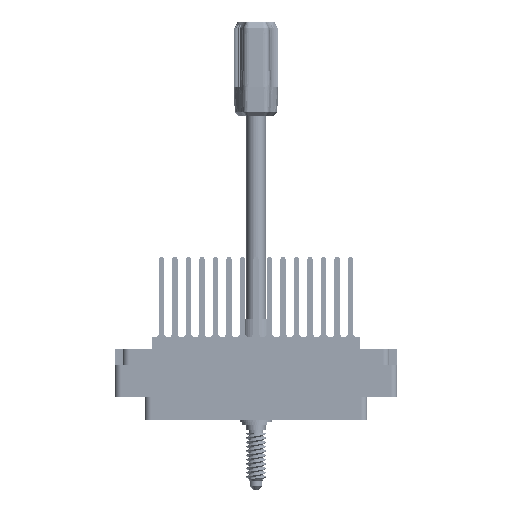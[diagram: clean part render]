
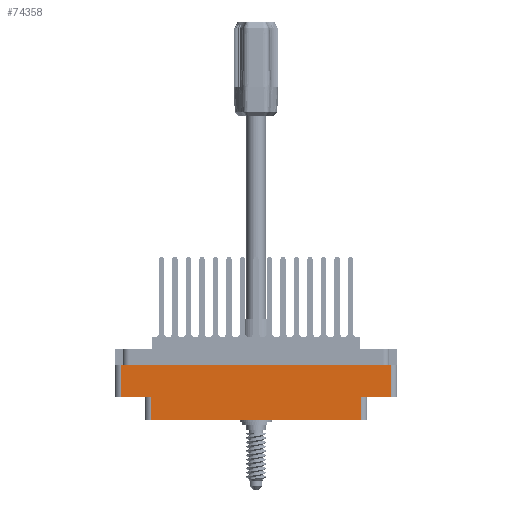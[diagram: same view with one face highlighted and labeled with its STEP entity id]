
A CAD part, front view. The second image highlights one B-rep face of the part: STEP entity #74358.
In plain terms, the highlighted planar face has unit normal (0, -1, 0).
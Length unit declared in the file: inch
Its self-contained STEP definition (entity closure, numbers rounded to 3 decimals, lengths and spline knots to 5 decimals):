
#1422 = CARTESIAN_POINT ( 'NONE',  ( -1.359, -0.617, -0.798 ) ) ;
#1529 = CARTESIAN_POINT ( 'NONE',  ( -1.359, -0.617, -0.798 ) ) ;
#1638 = CARTESIAN_POINT ( 'NONE',  ( 1.297, -0.617, -0.274 ) ) ;
#1776 = CARTESIAN_POINT ( 'NONE',  ( -1.297, -0.617, -0.274 ) ) ;
#3254 = ORIENTED_EDGE ( 'NONE', *, *, #56275, .T. ) ;
#5570 = DIRECTION ( 'NONE',  ( 1., 0., 0. ) ) ;
#8130 = LINE ( 'NONE', #80996, #48906 ) ;
#8278 = CARTESIAN_POINT ( 'NONE',  ( -1.006, -0.617, -0.798 ) ) ;
#8381 = VERTEX_POINT ( 'NONE', #32250 ) ;
#8851 = FACE_OUTER_BOUND ( 'NONE', #68375, .T. ) ;
#10698 = CARTESIAN_POINT ( 'NONE',  ( -1.006, -0.617, -0.578 ) ) ;
#11979 = DIRECTION ( 'NONE',  ( 1., 0., 0. ) ) ;
#14887 = VERTEX_POINT ( 'NONE', #80019 ) ;
#17351 = EDGE_CURVE ( 'NONE', #64329, #26004, #29253, .T. ) ;
#18496 = ORIENTED_EDGE ( 'NONE', *, *, #59542, .T. ) ;
#20173 = CARTESIAN_POINT ( 'NONE',  ( -1.006, -0.617, -0.798 ) ) ;
#21833 = EDGE_CURVE ( 'NONE', #33005, #61526, #42912, .T. ) ;
#21993 = DIRECTION ( 'NONE',  ( 0., 0., -1. ) ) ;
#25161 = CARTESIAN_POINT ( 'NONE',  ( 1.297, -0.617, -0.798 ) ) ;
#26004 = VERTEX_POINT ( 'NONE', #20173 ) ;
#26287 = ORIENTED_EDGE ( 'NONE', *, *, #17351, .T. ) ;
#26565 = CARTESIAN_POINT ( 'NONE',  ( -1.297, -0.617, -0.798 ) ) ;
#27351 = VECTOR ( 'NONE', #28329, 39.37008 ) ;
#28329 = DIRECTION ( 'NONE',  ( 1., 0., 0. ) ) ;
#28855 = DIRECTION ( 'NONE',  ( -1., 0., 0. ) ) ;
#29085 = ORIENTED_EDGE ( 'NONE', *, *, #21833, .T. ) ;
#29253 = LINE ( 'NONE', #8278, #61905 ) ;
#32250 = CARTESIAN_POINT ( 'NONE',  ( 1.297, -0.617, -0.578 ) ) ;
#33005 = VERTEX_POINT ( 'NONE', #1776 ) ;
#33332 = ORIENTED_EDGE ( 'NONE', *, *, #72745, .F. ) ;
#34723 = LINE ( 'NONE', #50304, #76542 ) ;
#34889 = AXIS2_PLACEMENT_3D ( 'NONE', #1422, #72163, #46978 ) ;
#36782 = ORIENTED_EDGE ( 'NONE', *, *, #84070, .F. ) ;
#38743 = CARTESIAN_POINT ( 'NONE',  ( 0., -0.617, -0.578 ) ) ;
#38840 = VECTOR ( 'NONE', #47336, 39.37008 ) ;
#41180 = VERTEX_POINT ( 'NONE', #1638 ) ;
#41368 = LINE ( 'NONE', #25161, #55709 ) ;
#42912 = LINE ( 'NONE', #26565, #38840 ) ;
#44275 = ORIENTED_EDGE ( 'NONE', *, *, #66893, .T. ) ;
#46978 = DIRECTION ( 'NONE',  ( 0., 0., -1. ) ) ;
#47292 = CARTESIAN_POINT ( 'NONE',  ( -1.297, -0.617, -0.578 ) ) ;
#47336 = DIRECTION ( 'NONE',  ( 0., 0., -1. ) ) ;
#48906 = VECTOR ( 'NONE', #28855, 39.37008 ) ;
#50304 = CARTESIAN_POINT ( 'NONE',  ( 0., -0.617, -0.274 ) ) ;
#50548 = VECTOR ( 'NONE', #77657, 39.37008 ) ;
#50859 = VECTOR ( 'NONE', #11979, 39.37008 ) ;
#52581 = LINE ( 'NONE', #59383, #50548 ) ;
#52699 = PLANE ( 'NONE',  #34889 ) ;
#55709 = VECTOR ( 'NONE', #77277, 39.37008 ) ;
#56275 = EDGE_CURVE ( 'NONE', #61526, #64329, #63203, .T. ) ;
#59383 = CARTESIAN_POINT ( 'NONE',  ( 1.006, -0.617, -0.578 ) ) ;
#59542 = EDGE_CURVE ( 'NONE', #8381, #41180, #41368, .T. ) ;
#60954 = ORIENTED_EDGE ( 'NONE', *, *, #68743, .T. ) ;
#61526 = VERTEX_POINT ( 'NONE', #47292 ) ;
#61905 = VECTOR ( 'NONE', #21993, 39.37008 ) ;
#63203 = LINE ( 'NONE', #38743, #50859 ) ;
#64329 = VERTEX_POINT ( 'NONE', #10698 ) ;
#66893 = EDGE_CURVE ( 'NONE', #26004, #73122, #75341, .T. ) ;
#68375 = EDGE_LOOP ( 'NONE', ( #3254, #26287, #44275, #60954, #36782, #18496, #33332, #29085 ) ) ;
#68743 = EDGE_CURVE ( 'NONE', #73122, #14887, #52581, .T. ) ;
#72163 = DIRECTION ( 'NONE',  ( 0., -1., 0. ) ) ;
#72745 = EDGE_CURVE ( 'NONE', #33005, #41180, #34723, .T. ) ;
#73122 = VERTEX_POINT ( 'NONE', #75552 ) ;
#74358 = ADVANCED_FACE ( 'NONE', ( #8851 ), #52699, .T. ) ;
#75341 = LINE ( 'NONE', #1529, #27351 ) ;
#75552 = CARTESIAN_POINT ( 'NONE',  ( 1.006, -0.617, -0.798 ) ) ;
#76542 = VECTOR ( 'NONE', #5570, 39.37008 ) ;
#77277 = DIRECTION ( 'NONE',  ( 0., 0., 1. ) ) ;
#77657 = DIRECTION ( 'NONE',  ( 0., 0., 1. ) ) ;
#80019 = CARTESIAN_POINT ( 'NONE',  ( 1.006, -0.617, -0.578 ) ) ;
#80996 = CARTESIAN_POINT ( 'NONE',  ( 0., -0.617, -0.578 ) ) ;
#84070 = EDGE_CURVE ( 'NONE', #8381, #14887, #8130, .T. ) ;
